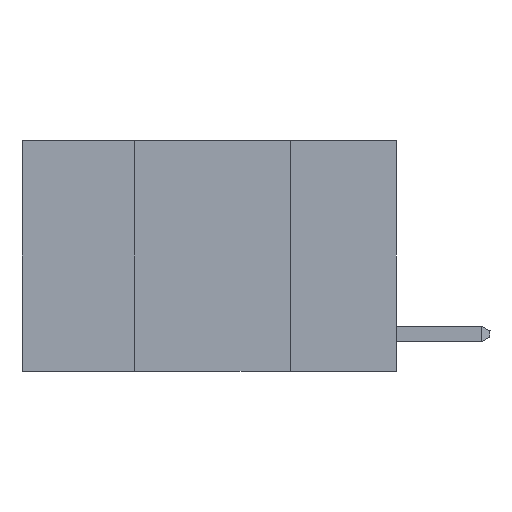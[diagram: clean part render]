
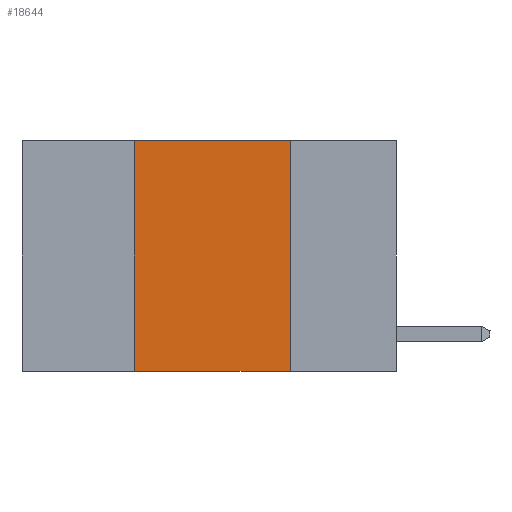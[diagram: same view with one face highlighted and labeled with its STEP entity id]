
A CAD part, left-side view. The second image highlights one B-rep face of the part: STEP entity #18644.
In plain terms, the highlighted planar face has unit normal (-1, 0, 0).
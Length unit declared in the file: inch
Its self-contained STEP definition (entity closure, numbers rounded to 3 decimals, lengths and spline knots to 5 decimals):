
#117 = VECTOR ( 'NONE', #14541, 39.37008 ) ;
#579 = DIRECTION ( 'NONE',  ( 0., 0., -1. ) ) ;
#763 = CARTESIAN_POINT ( 'NONE',  ( 0., 0.6, 0. ) ) ;
#803 = CARTESIAN_POINT ( 'NONE',  ( 0., 0.42, -0.37 ) ) ;
#977 = ORIENTED_EDGE ( 'NONE', *, *, #27245, .F. ) ;
#4181 = LINE ( 'NONE', #15026, #26397 ) ;
#4275 = VERTEX_POINT ( 'NONE', #23245 ) ;
#6241 = DIRECTION ( 'NONE',  ( 0., 0., 1. ) ) ;
#6493 = DIRECTION ( 'NONE',  ( 0., 0., -1. ) ) ;
#7674 = VERTEX_POINT ( 'NONE', #13644 ) ;
#8066 = VERTEX_POINT ( 'NONE', #9640 ) ;
#9251 = EDGE_CURVE ( 'NONE', #11626, #8066, #26654, .T. ) ;
#9640 = CARTESIAN_POINT ( 'NONE',  ( 0., 0.42, 0. ) ) ;
#9641 = AXIS2_PLACEMENT_3D ( 'NONE', #763, #11688, #579 ) ;
#11420 = LINE ( 'NONE', #19620, #16471 ) ;
#11462 = EDGE_LOOP ( 'NONE', ( #18556, #977, #20351, #17800 ) ) ;
#11626 = VERTEX_POINT ( 'NONE', #803 ) ;
#11688 = DIRECTION ( 'NONE',  ( 1., 0., 0. ) ) ;
#11841 = VECTOR ( 'NONE', #6241, 39.37008 ) ;
#12432 = EDGE_CURVE ( 'NONE', #7674, #4275, #4181, .T. ) ;
#13644 = CARTESIAN_POINT ( 'NONE',  ( 0., 0.17, 0. ) ) ;
#14541 = DIRECTION ( 'NONE',  ( 0., -1., 0. ) ) ;
#15026 = CARTESIAN_POINT ( 'NONE',  ( 0., 0.17, 0. ) ) ;
#16471 = VECTOR ( 'NONE', #26232, 39.37008 ) ;
#17800 = ORIENTED_EDGE ( 'NONE', *, *, #21013, .T. ) ;
#18556 = ORIENTED_EDGE ( 'NONE', *, *, #12432, .F. ) ;
#18644 = ADVANCED_FACE ( 'NONE', ( #27219 ), #22139, .F. ) ;
#19298 = LINE ( 'NONE', #25108, #117 ) ;
#19620 = CARTESIAN_POINT ( 'NONE',  ( 0., 0.6, 0. ) ) ;
#20351 = ORIENTED_EDGE ( 'NONE', *, *, #9251, .F. ) ;
#20530 = CARTESIAN_POINT ( 'NONE',  ( 0., 0.42, 0. ) ) ;
#21013 = EDGE_CURVE ( 'NONE', #11626, #4275, #19298, .T. ) ;
#22139 = PLANE ( 'NONE',  #9641 ) ;
#23245 = CARTESIAN_POINT ( 'NONE',  ( 0., 0.17, -0.37 ) ) ;
#25108 = CARTESIAN_POINT ( 'NONE',  ( 0., 0.6, -0.37 ) ) ;
#26232 = DIRECTION ( 'NONE',  ( 0., -1., 0. ) ) ;
#26397 = VECTOR ( 'NONE', #6493, 39.37008 ) ;
#26654 = LINE ( 'NONE', #20530, #11841 ) ;
#27219 = FACE_OUTER_BOUND ( 'NONE', #11462, .T. ) ;
#27245 = EDGE_CURVE ( 'NONE', #8066, #7674, #11420, .T. ) ;
